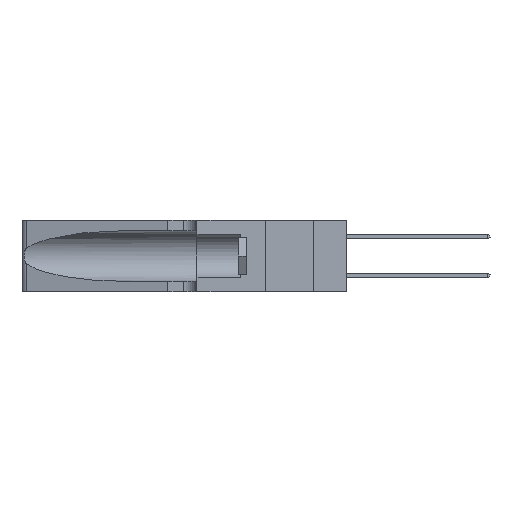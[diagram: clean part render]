
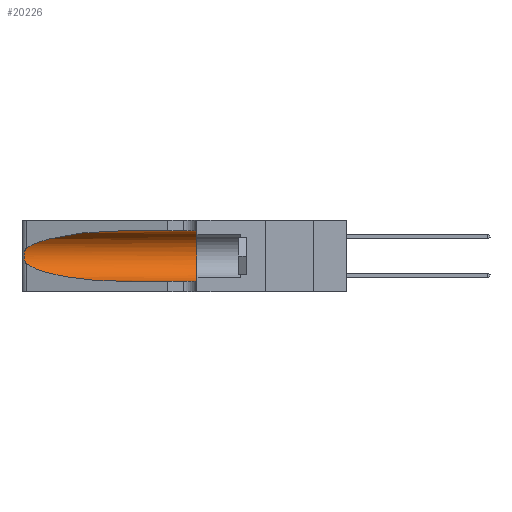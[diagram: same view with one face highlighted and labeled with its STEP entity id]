
A CAD part, left-side view. The second image highlights one B-rep face of the part: STEP entity #20226.
In plain terms, the highlighted cylindrical face has radius 3.308 mm (diameter 6.617 mm), a partial arc.
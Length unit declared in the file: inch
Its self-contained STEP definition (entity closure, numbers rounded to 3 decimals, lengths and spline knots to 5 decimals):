
#652 =( BOUNDED_CURVE ( )  B_SPLINE_CURVE ( 3, ( #18686, #21001, #6915, #4701 ),
 .UNSPECIFIED., .F., .F. ) 
 B_SPLINE_CURVE_WITH_KNOTS ( ( 4, 4 ),
 ( 3.44316, 4.71239 ),
 .UNSPECIFIED. ) 
 CURVE ( )  GEOMETRIC_REPRESENTATION_ITEM ( )  RATIONAL_B_SPLINE_CURVE ( ( 1., 0.87, 0.87, 1. ) ) 
 REPRESENTATION_ITEM ( '' )  );
#1763 = CARTESIAN_POINT ( 'NONE',  ( 0.25639, 1.23184, 0.21858 ) ) ;
#2266 = EDGE_CURVE ( 'NONE', #22461, #23343, #17970, .T. ) ;
#2437 = VECTOR ( 'NONE', #5876, 39.37008 ) ;
#2573 = CARTESIAN_POINT ( 'NONE',  ( 0.25487, 1.22718, 0.22369 ) ) ;
#3330 = DIRECTION ( 'NONE',  ( 0., -1., 0. ) ) ;
#3777 = CARTESIAN_POINT ( 'NONE',  ( 0.25555, 1.22994, 0.2215 ) ) ;
#3932 = CARTESIAN_POINT ( 'NONE',  ( 0.1305, 1.61858, 0.31525 ) ) ;
#4701 = CARTESIAN_POINT ( 'NONE',  ( 0.1305, 0.72297, 0.05475 ) ) ;
#5490 = VECTOR ( 'NONE', #3330, 39.37008 ) ;
#5876 = DIRECTION ( 'NONE',  ( 0., -1., 0. ) ) ;
#6152 = CARTESIAN_POINT ( 'NONE',  ( 0.1305, 0.72297, 0.31525 ) ) ;
#6915 = CARTESIAN_POINT ( 'NONE',  ( 0.18966, 0.96281, 0.05475 ) ) ;
#6916 = ORIENTED_EDGE ( 'NONE', *, *, #17999, .T. ) ;
#7377 = CARTESIAN_POINT ( 'NONE',  ( 0.1305, 1.61858, 0.185 ) ) ;
#7391 = EDGE_CURVE ( 'NONE', #23343, #9269, #20259, .T. ) ;
#7675 = CARTESIAN_POINT ( 'NONE',  ( 0.26075, 1.23896, 0.178 ) ) ;
#7769 = CARTESIAN_POINT ( 'NONE',  ( 0.25854, 1.2359, 0.20912 ) ) ;
#8938 = VERTEX_POINT ( 'NONE', #22822 ) ;
#9074 = DIRECTION ( 'NONE',  ( 0., -1., 0. ) ) ;
#9269 = VERTEX_POINT ( 'NONE', #25724 ) ;
#9365 = AXIS2_PLACEMENT_3D ( 'NONE', #7377, #9074, #21537 ) ;
#9554 = CARTESIAN_POINT ( 'NONE',  ( 0.18966, 0.96281, 0.31525 ) ) ;
#10088 = CARTESIAN_POINT ( 'NONE',  ( 0.25789, 1.23486, 0.15765 ) ) ;
#10461 = FACE_OUTER_BOUND ( 'NONE', #10785, .T. ) ;
#10785 = EDGE_LOOP ( 'NONE', ( #10918, #11570, #13454, #6916, #16072, #22774 ) ) ;
#10903 = CARTESIAN_POINT ( 'NONE',  ( 0.1305, 0.35, 0.185 ) ) ;
#10918 = ORIENTED_EDGE ( 'NONE', *, *, #2266, .T. ) ;
#11570 = ORIENTED_EDGE ( 'NONE', *, *, #7391, .T. ) ;
#11745 = CARTESIAN_POINT ( 'NONE',  ( 0.25487, 1.22718, 0.22369 ) ) ;
#11933 = CARTESIAN_POINT ( 'NONE',  ( 0.25639, 1.23186, 0.15144 ) ) ;
#12045 = CARTESIAN_POINT ( 'NONE',  ( 0.1305, 0.72297, 0.31525 ) ) ;
#12176 = CARTESIAN_POINT ( 'NONE',  ( 0.25487, 1.22718, 0.22369 ) ) ;
#12187 = VERTEX_POINT ( 'NONE', #15664 ) ;
#12407 = AXIS2_PLACEMENT_3D ( 'NONE', #10903, #20892, #23004 ) ;
#13210 = LINE ( 'NONE', #3932, #2437 ) ;
#13454 = ORIENTED_EDGE ( 'NONE', *, *, #18472, .T. ) ;
#14115 = CARTESIAN_POINT ( 'NONE',  ( 0.2373, 1.15595, 0.28018 ) ) ;
#15664 = CARTESIAN_POINT ( 'NONE',  ( 0.1305, 0.35, 0.31525 ) ) ;
#16072 = ORIENTED_EDGE ( 'NONE', *, *, #20767, .F. ) ;
#16383 = EDGE_CURVE ( 'NONE', #22461, #12187, #13210, .T. ) ;
#16759 = CIRCLE ( 'NONE', #12407, 0.13025 ) ;
#16850 = VERTEX_POINT ( 'NONE', #18048 ) ;
#17857 = CARTESIAN_POINT ( 'NONE',  ( 0.26075, 1.23896, 0.19203 ) ) ;
#17970 =( BOUNDED_CURVE ( )  B_SPLINE_CURVE ( 3, ( #6152, #9554, #14115, #12176 ),
 .UNSPECIFIED., .F., .F. ) 
 B_SPLINE_CURVE_WITH_KNOTS ( ( 4, 4 ),
 ( 1.5708, 2.84003 ),
 .UNSPECIFIED. ) 
 CURVE ( )  GEOMETRIC_REPRESENTATION_ITEM ( )  RATIONAL_B_SPLINE_CURVE ( ( 1., 0.87, 0.87, 1. ) ) 
 REPRESENTATION_ITEM ( '' )  );
#17999 = EDGE_CURVE ( 'NONE', #8938, #16850, #23830, .T. ) ;
#18048 = CARTESIAN_POINT ( 'NONE',  ( 0.1305, 0.35, 0.05475 ) ) ;
#18118 = CARTESIAN_POINT ( 'NONE',  ( 0.26018, 1.23835, 0.19895 ) ) ;
#18472 = EDGE_CURVE ( 'NONE', #9269, #8938, #652, .T. ) ;
#18686 = CARTESIAN_POINT ( 'NONE',  ( 0.25487, 1.22718, 0.14631 ) ) ;
#19292 = CYLINDRICAL_SURFACE ( 'NONE', #9365, 0.13025 ) ;
#19886 = CARTESIAN_POINT ( 'NONE',  ( 0.25487, 1.22718, 0.14631 ) ) ;
#19973 = CARTESIAN_POINT ( 'NONE',  ( 0.25555, 1.22993, 0.14849 ) ) ;
#20226 = ADVANCED_FACE ( 'NONE', ( #10461 ), #19292, .F. ) ;
#20259 = B_SPLINE_CURVE_WITH_KNOTS ( 'NONE', 3,
 ( #11745, #3777, #1763, #21844, #7769, #18118, #17857, #7675, #24215, #21938, #10088, #11933, #19973, #19886 ),
 .UNSPECIFIED., .F., .F.,
 ( 4, 2, 2, 2, 2, 2, 4 ),
 ( 0., 0.00027, 0.00053, 0.00107, 0.0016, 0.00187, 0.00214 ),
 .UNSPECIFIED. ) ;
#20767 = EDGE_CURVE ( 'NONE', #12187, #16850, #16759, .T. ) ;
#20892 = DIRECTION ( 'NONE',  ( 0., 1., 0. ) ) ;
#21001 = CARTESIAN_POINT ( 'NONE',  ( 0.2373, 1.15595, 0.08982 ) ) ;
#21537 = DIRECTION ( 'NONE',  ( 0., 0., -1. ) ) ;
#21844 = CARTESIAN_POINT ( 'NONE',  ( 0.25787, 1.23484, 0.2124 ) ) ;
#21938 = CARTESIAN_POINT ( 'NONE',  ( 0.25856, 1.23593, 0.16098 ) ) ;
#22461 = VERTEX_POINT ( 'NONE', #12045 ) ;
#22774 = ORIENTED_EDGE ( 'NONE', *, *, #16383, .F. ) ;
#22822 = CARTESIAN_POINT ( 'NONE',  ( 0.1305, 0.72297, 0.05475 ) ) ;
#23004 = DIRECTION ( 'NONE',  ( 0., 0., 1. ) ) ;
#23343 = VERTEX_POINT ( 'NONE', #2573 ) ;
#23830 = LINE ( 'NONE', #25680, #5490 ) ;
#24215 = CARTESIAN_POINT ( 'NONE',  ( 0.26017, 1.23833, 0.17102 ) ) ;
#25680 = CARTESIAN_POINT ( 'NONE',  ( 0.1305, 1.61858, 0.05475 ) ) ;
#25724 = CARTESIAN_POINT ( 'NONE',  ( 0.25487, 1.22718, 0.14631 ) ) ;
